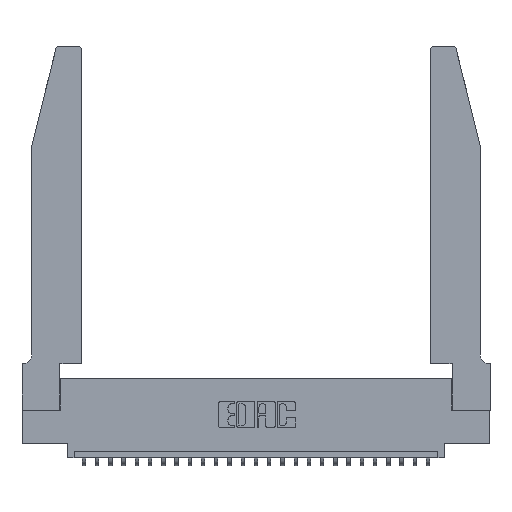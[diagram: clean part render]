
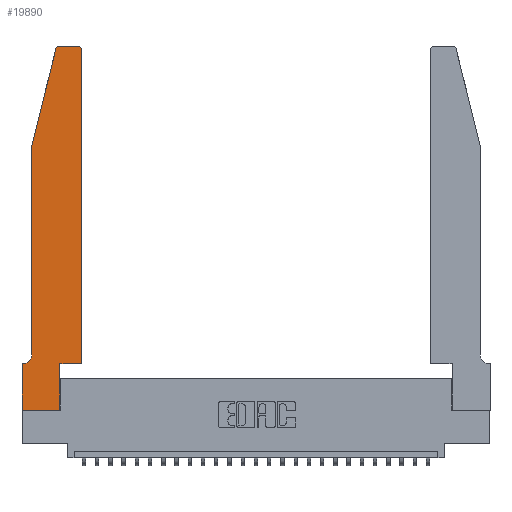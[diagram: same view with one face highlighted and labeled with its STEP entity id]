
A CAD part, top view. The second image highlights one B-rep face of the part: STEP entity #19890.
In plain terms, the highlighted planar face has unit normal (0, 0, 1).
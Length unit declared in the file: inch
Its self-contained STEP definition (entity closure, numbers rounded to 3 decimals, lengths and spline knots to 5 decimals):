
#41 = DIRECTION ( 'NONE',  ( -1., 0., 0. ) ) ;
#246 = DIRECTION ( 'NONE',  ( 1., 0., 0. ) ) ;
#269 = CARTESIAN_POINT ( 'NONE',  ( 0.0055, 0.35, 0.37 ) ) ;
#918 = CARTESIAN_POINT ( 'NONE',  ( 0.284, 2.75, 0.37 ) ) ;
#921 = LINE ( 'NONE', #18934, #17746 ) ;
#969 = VECTOR ( 'NONE', #25507, 39.37008 ) ;
#1094 = VECTOR ( 'NONE', #19807, 39.37008 ) ;
#1146 = VERTEX_POINT ( 'NONE', #1380 ) ;
#1192 = LINE ( 'NONE', #10747, #1518 ) ;
#1380 = CARTESIAN_POINT ( 'NONE',  ( 0., 0.35, 0.37 ) ) ;
#1518 = VECTOR ( 'NONE', #12889, 39.37008 ) ;
#1679 = EDGE_CURVE ( 'NONE', #26234, #2776, #6716, .T. ) ;
#1690 = EDGE_CURVE ( 'NONE', #1146, #17641, #5401, .T. ) ;
#2549 = DIRECTION ( 'NONE',  ( 0., -1., 0. ) ) ;
#2776 = VERTEX_POINT ( 'NONE', #918 ) ;
#2886 = CARTESIAN_POINT ( 'NONE',  ( 0.2605, 2.75, 0.37 ) ) ;
#2988 = ORIENTED_EDGE ( 'NONE', *, *, #25770, .T. ) ;
#3363 = VECTOR ( 'NONE', #7524, 39.37008 ) ;
#4229 = ORIENTED_EDGE ( 'NONE', *, *, #1679, .T. ) ;
#4365 = VERTEX_POINT ( 'NONE', #13020 ) ;
#4718 = VERTEX_POINT ( 'NONE', #8854 ) ;
#5401 = LINE ( 'NONE', #11257, #21504 ) ;
#5815 = VERTEX_POINT ( 'NONE', #8563 ) ;
#5882 = CARTESIAN_POINT ( 'NONE',  ( 0.25487, 2.72718, 0.37 ) ) ;
#5914 = DIRECTION ( 'NONE',  ( 0., 0., 1. ) ) ;
#6175 = ORIENTED_EDGE ( 'NONE', *, *, #21159, .T. ) ;
#6609 = DIRECTION ( 'NONE',  ( 1., 0., 0. ) ) ;
#6716 = LINE ( 'NONE', #2886, #1094 ) ;
#7084 = VERTEX_POINT ( 'NONE', #20491 ) ;
#7524 = DIRECTION ( 'NONE',  ( 0., 1., 0. ) ) ;
#8399 = CIRCLE ( 'NONE', #15811, 0.07 ) ;
#8563 = CARTESIAN_POINT ( 'NONE',  ( 0.0755, 0.42, 0.37 ) ) ;
#8854 = CARTESIAN_POINT ( 'NONE',  ( 0.2865, 0., 0.37 ) ) ;
#9315 = ORIENTED_EDGE ( 'NONE', *, *, #24061, .T. ) ;
#9469 = DIRECTION ( 'NONE',  ( 1., 0., 0. ) ) ;
#9681 = EDGE_CURVE ( 'NONE', #2776, #20323, #21545, .T. ) ;
#10364 = ORIENTED_EDGE ( 'NONE', *, *, #9681, .T. ) ;
#10399 = CARTESIAN_POINT ( 'NONE',  ( 0.0755, 2., 0.37 ) ) ;
#10747 = CARTESIAN_POINT ( 'NONE',  ( 0.0755, 2., 0.37 ) ) ;
#10940 = DIRECTION ( 'NONE',  ( 0., 0., 1. ) ) ;
#11257 = CARTESIAN_POINT ( 'NONE',  ( 0., 0., 0.37 ) ) ;
#11981 = DIRECTION ( 'NONE',  ( -1., 0., 0. ) ) ;
#12041 = VERTEX_POINT ( 'NONE', #26610 ) ;
#12607 = CARTESIAN_POINT ( 'NONE',  ( 0.0755, 0.35, 0.37 ) ) ;
#12850 = LINE ( 'NONE', #15176, #969 ) ;
#12889 = DIRECTION ( 'NONE',  ( -0.239, -0.971, 0. ) ) ;
#12984 = PLANE ( 'NONE',  #17403 ) ;
#13020 = CARTESIAN_POINT ( 'NONE',  ( 0.2865, 0.35, 0.37 ) ) ;
#13892 = CARTESIAN_POINT ( 'NONE',  ( 0.2865, 0.35, 0.37 ) ) ;
#14621 = VECTOR ( 'NONE', #41, 39.37008 ) ;
#14650 = ORIENTED_EDGE ( 'NONE', *, *, #1690, .T. ) ;
#15176 = CARTESIAN_POINT ( 'NONE',  ( 0.4505, 0.35, 0.37 ) ) ;
#15811 = AXIS2_PLACEMENT_3D ( 'NONE', #16309, #22649, #11981 ) ;
#16309 = CARTESIAN_POINT ( 'NONE',  ( 0.0055, 0.42, 0.37 ) ) ;
#16583 = DIRECTION ( 'NONE',  ( 1., 0., 0. ) ) ;
#17031 = CARTESIAN_POINT ( 'NONE',  ( 0., 0., 0.37 ) ) ;
#17282 = VERTEX_POINT ( 'NONE', #269 ) ;
#17403 = AXIS2_PLACEMENT_3D ( 'NONE', #25872, #10940, #246 ) ;
#17641 = VERTEX_POINT ( 'NONE', #17031 ) ;
#17746 = VECTOR ( 'NONE', #6609, 39.37008 ) ;
#18572 = EDGE_CURVE ( 'NONE', #17282, #1146, #27161, .T. ) ;
#18831 = FACE_OUTER_BOUND ( 'NONE', #26759, .T. ) ;
#18858 = LINE ( 'NONE', #21690, #23114 ) ;
#18934 = CARTESIAN_POINT ( 'NONE',  ( 0.4505, 0.35, 0.37 ) ) ;
#19152 = ORIENTED_EDGE ( 'NONE', *, *, #22278, .T. ) ;
#19533 = DIRECTION ( 'NONE',  ( 0., -1., 0. ) ) ;
#19775 = CARTESIAN_POINT ( 'NONE',  ( 0.4205, 2.72, 0.37 ) ) ;
#19807 = DIRECTION ( 'NONE',  ( -1., 0., 0. ) ) ;
#19890 = ADVANCED_FACE ( 'NONE', ( #18831 ), #12984, .T. ) ;
#20323 = VERTEX_POINT ( 'NONE', #5882 ) ;
#20394 = CARTESIAN_POINT ( 'NONE',  ( 0., 0., 0.37 ) ) ;
#20491 = CARTESIAN_POINT ( 'NONE',  ( 0.4505, 2.72, 0.37 ) ) ;
#20675 = LINE ( 'NONE', #20394, #23618 ) ;
#20721 = ORIENTED_EDGE ( 'NONE', *, *, #26995, .T. ) ;
#20803 = LINE ( 'NONE', #13892, #3363 ) ;
#20921 = CIRCLE ( 'NONE', #26191, 0.03 ) ;
#21159 = EDGE_CURVE ( 'NONE', #22910, #5815, #18858, .T. ) ;
#21476 = EDGE_CURVE ( 'NONE', #4718, #4365, #20803, .T. ) ;
#21504 = VECTOR ( 'NONE', #19533, 39.37008 ) ;
#21545 = CIRCLE ( 'NONE', #25324, 0.03 ) ;
#21690 = CARTESIAN_POINT ( 'NONE',  ( 0.0755, 2., 0.37 ) ) ;
#21793 = ORIENTED_EDGE ( 'NONE', *, *, #23283, .T. ) ;
#22278 = EDGE_CURVE ( 'NONE', #12041, #7084, #12850, .T. ) ;
#22649 = DIRECTION ( 'NONE',  ( 0., 0., -1. ) ) ;
#22687 = ORIENTED_EDGE ( 'NONE', *, *, #18572, .T. ) ;
#22910 = VERTEX_POINT ( 'NONE', #10399 ) ;
#23114 = VECTOR ( 'NONE', #2549, 39.37008 ) ;
#23283 = EDGE_CURVE ( 'NONE', #17641, #4718, #20675, .T. ) ;
#23502 = ORIENTED_EDGE ( 'NONE', *, *, #25520, .T. ) ;
#23618 = VECTOR ( 'NONE', #24343, 39.37008 ) ;
#23907 = DIRECTION ( 'NONE',  ( 0., 0., 1. ) ) ;
#24061 = EDGE_CURVE ( 'NONE', #20323, #22910, #1192, .T. ) ;
#24343 = DIRECTION ( 'NONE',  ( 1., 0., 0. ) ) ;
#24851 = CARTESIAN_POINT ( 'NONE',  ( 0.284, 2.72, 0.37 ) ) ;
#25265 = CARTESIAN_POINT ( 'NONE',  ( 0.4205, 2.75, 0.37 ) ) ;
#25324 = AXIS2_PLACEMENT_3D ( 'NONE', #24851, #5914, #16583 ) ;
#25507 = DIRECTION ( 'NONE',  ( 0., 1., 0. ) ) ;
#25520 = EDGE_CURVE ( 'NONE', #5815, #17282, #8399, .T. ) ;
#25770 = EDGE_CURVE ( 'NONE', #7084, #26234, #20921, .T. ) ;
#25872 = CARTESIAN_POINT ( 'NONE',  ( 0., 0.35, 0.37 ) ) ;
#26191 = AXIS2_PLACEMENT_3D ( 'NONE', #19775, #23907, #9469 ) ;
#26234 = VERTEX_POINT ( 'NONE', #25265 ) ;
#26568 = ORIENTED_EDGE ( 'NONE', *, *, #21476, .T. ) ;
#26610 = CARTESIAN_POINT ( 'NONE',  ( 0.4505, 0.35, 0.37 ) ) ;
#26759 = EDGE_LOOP ( 'NONE', ( #4229, #10364, #9315, #6175, #23502, #22687, #14650, #21793, #26568, #20721, #19152, #2988 ) ) ;
#26995 = EDGE_CURVE ( 'NONE', #4365, #12041, #921, .T. ) ;
#27161 = LINE ( 'NONE', #12607, #14621 ) ;
